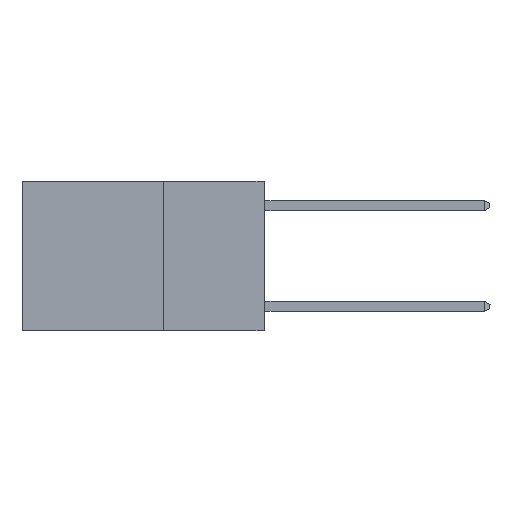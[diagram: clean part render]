
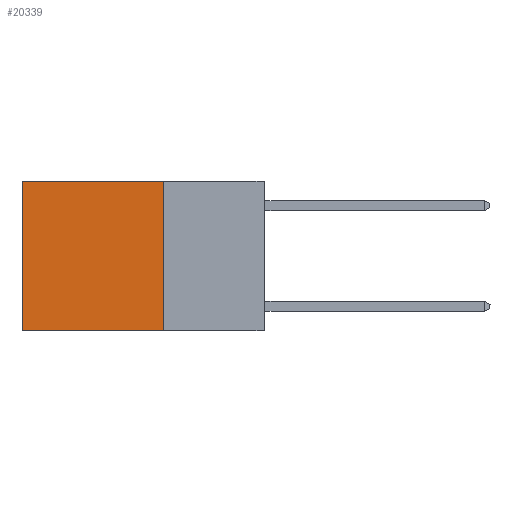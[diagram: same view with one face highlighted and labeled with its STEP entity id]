
A CAD part, left-side view. The second image highlights one B-rep face of the part: STEP entity #20339.
In plain terms, the highlighted planar face has unit normal (-1, 0, 0).
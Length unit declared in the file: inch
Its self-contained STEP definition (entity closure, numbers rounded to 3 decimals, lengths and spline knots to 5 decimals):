
#651 = DIRECTION ( 'NONE',  ( 0., 0., -1. ) ) ;
#778 = VERTEX_POINT ( 'NONE', #5131 ) ;
#1028 = LINE ( 'NONE', #14783, #12777 ) ;
#1493 = CARTESIAN_POINT ( 'NONE',  ( 0.2625, 0.6, -0.37 ) ) ;
#1917 = ORIENTED_EDGE ( 'NONE', *, *, #17540, .T. ) ;
#2010 = CARTESIAN_POINT ( 'NONE',  ( 0.2625, 0.25, -0.37 ) ) ;
#2399 = VECTOR ( 'NONE', #651, 39.37008 ) ;
#2881 = DIRECTION ( 'NONE',  ( 1., 0., 0. ) ) ;
#2887 = LINE ( 'NONE', #7233, #6628 ) ;
#3500 = CARTESIAN_POINT ( 'NONE',  ( 0.2625, 0.6, 0. ) ) ;
#4933 = EDGE_CURVE ( 'NONE', #778, #7431, #1028, .T. ) ;
#5131 = CARTESIAN_POINT ( 'NONE',  ( 0.2625, 0.25, 0. ) ) ;
#6628 = VECTOR ( 'NONE', #8759, 39.37008 ) ;
#6900 = DIRECTION ( 'NONE',  ( 0., 1., 0. ) ) ;
#7233 = CARTESIAN_POINT ( 'NONE',  ( 0.2625, 0.25, 0. ) ) ;
#7431 = VERTEX_POINT ( 'NONE', #11726 ) ;
#7546 = PLANE ( 'NONE',  #12265 ) ;
#7827 = CARTESIAN_POINT ( 'NONE',  ( 0.2625, 0.25, 0. ) ) ;
#8276 = VERTEX_POINT ( 'NONE', #12245 ) ;
#8331 = FACE_OUTER_BOUND ( 'NONE', #9467, .T. ) ;
#8568 = ORIENTED_EDGE ( 'NONE', *, *, #4933, .F. ) ;
#8759 = DIRECTION ( 'NONE',  ( 0., 1., 0. ) ) ;
#9467 = EDGE_LOOP ( 'NONE', ( #1917, #16157, #8568, #11695 ) ) ;
#9777 = LINE ( 'NONE', #2010, #18314 ) ;
#11400 = EDGE_CURVE ( 'NONE', #7431, #20389, #9777, .T. ) ;
#11695 = ORIENTED_EDGE ( 'NONE', *, *, #19492, .T. ) ;
#11726 = CARTESIAN_POINT ( 'NONE',  ( 0.2625, 0.25, -0.37 ) ) ;
#12245 = CARTESIAN_POINT ( 'NONE',  ( 0.2625, 0.6, 0. ) ) ;
#12265 = AXIS2_PLACEMENT_3D ( 'NONE', #7827, #2881, #15817 ) ;
#12777 = VECTOR ( 'NONE', #13040, 39.37008 ) ;
#13040 = DIRECTION ( 'NONE',  ( 0., 0., -1. ) ) ;
#14783 = CARTESIAN_POINT ( 'NONE',  ( 0.2625, 0.25, 0. ) ) ;
#15817 = DIRECTION ( 'NONE',  ( 0., 0., -1. ) ) ;
#16157 = ORIENTED_EDGE ( 'NONE', *, *, #11400, .F. ) ;
#17540 = EDGE_CURVE ( 'NONE', #8276, #20389, #19431, .T. ) ;
#18314 = VECTOR ( 'NONE', #6900, 39.37008 ) ;
#19431 = LINE ( 'NONE', #3500, #2399 ) ;
#19492 = EDGE_CURVE ( 'NONE', #778, #8276, #2887, .T. ) ;
#20339 = ADVANCED_FACE ( 'NONE', ( #8331 ), #7546, .F. ) ;
#20389 = VERTEX_POINT ( 'NONE', #1493 ) ;
